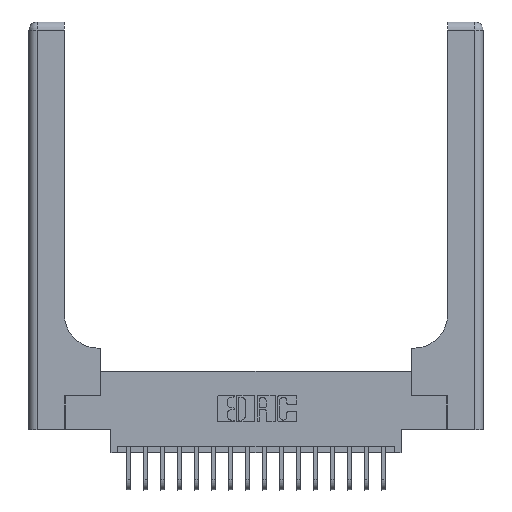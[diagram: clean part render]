
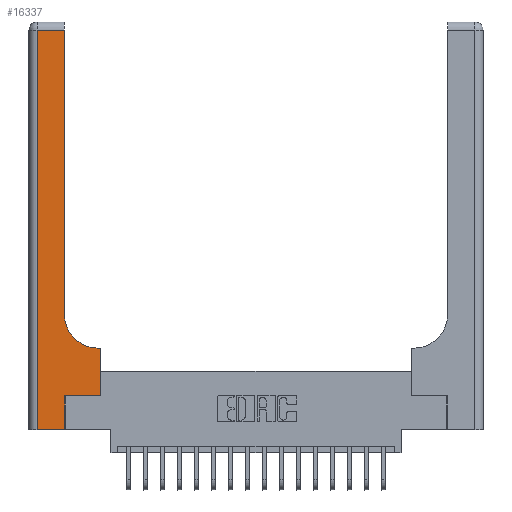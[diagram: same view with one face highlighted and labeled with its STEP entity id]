
A CAD part, top view. The second image highlights one B-rep face of the part: STEP entity #16337.
In plain terms, the highlighted planar face has unit normal (0, 0, 1).
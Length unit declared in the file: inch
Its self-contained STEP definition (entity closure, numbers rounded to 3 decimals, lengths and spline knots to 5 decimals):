
#122 = VECTOR ( 'NONE', #10542, 39.37008 ) ;
#211 = VERTEX_POINT ( 'NONE', #7665 ) ;
#335 = ORIENTED_EDGE ( 'NONE', *, *, #12892, .T. ) ;
#625 = DIRECTION ( 'NONE',  ( 0., 0., -1. ) ) ;
#673 = CARTESIAN_POINT ( 'NONE',  ( 0.265, 0., 0.37 ) ) ;
#1285 = EDGE_CURVE ( 'NONE', #3510, #17253, #9000, .T. ) ;
#1642 = AXIS2_PLACEMENT_3D ( 'NONE', #3078, #9773, #6152 ) ;
#1792 = LINE ( 'NONE', #16711, #8638 ) ;
#2145 = CARTESIAN_POINT ( 'NONE',  ( 0.528, 0.25, 0.37 ) ) ;
#2378 = LINE ( 'NONE', #12741, #17226 ) ;
#2574 = EDGE_CURVE ( 'NONE', #4467, #6856, #1792, .T. ) ;
#2607 = ORIENTED_EDGE ( 'NONE', *, *, #15406, .T. ) ;
#2895 = CARTESIAN_POINT ( 'NONE',  ( 0.265, 0.25, 0.37 ) ) ;
#3078 = CARTESIAN_POINT ( 'NONE',  ( 0.51, 0.85, 0.37 ) ) ;
#3272 = AXIS2_PLACEMENT_3D ( 'NONE', #15536, #625, #7302 ) ;
#3510 = VERTEX_POINT ( 'NONE', #9975 ) ;
#3886 = PLANE ( 'NONE',  #3272 ) ;
#3890 = ORIENTED_EDGE ( 'NONE', *, *, #6887, .T. ) ;
#4261 = CARTESIAN_POINT ( 'NONE',  ( 0.06, 3., 0.37 ) ) ;
#4445 = VERTEX_POINT ( 'NONE', #673 ) ;
#4467 = VERTEX_POINT ( 'NONE', #20370 ) ;
#5089 = DIRECTION ( 'NONE',  ( -1., 0., 0. ) ) ;
#6149 = CARTESIAN_POINT ( 'NONE',  ( 0.265, 0.25, 0.37 ) ) ;
#6152 = DIRECTION ( 'NONE',  ( 1., 0., 0. ) ) ;
#6190 = ORIENTED_EDGE ( 'NONE', *, *, #1285, .T. ) ;
#6856 = VERTEX_POINT ( 'NONE', #17533 ) ;
#6887 = EDGE_CURVE ( 'NONE', #6856, #15495, #11058, .T. ) ;
#7302 = DIRECTION ( 'NONE',  ( -1., 0., 0. ) ) ;
#7633 = VECTOR ( 'NONE', #19273, 39.37008 ) ;
#7665 = CARTESIAN_POINT ( 'NONE',  ( 0.26, 2.94, 0.37 ) ) ;
#7694 = LINE ( 'NONE', #16035, #7739 ) ;
#7739 = VECTOR ( 'NONE', #11409, 39.37008 ) ;
#7845 = ORIENTED_EDGE ( 'NONE', *, *, #11887, .T. ) ;
#8092 = DIRECTION ( 'NONE',  ( 0., 1., 0. ) ) ;
#8638 = VECTOR ( 'NONE', #5089, 39.37008 ) ;
#9000 = LINE ( 'NONE', #4261, #7633 ) ;
#9269 = FACE_OUTER_BOUND ( 'NONE', #9781, .T. ) ;
#9612 = VECTOR ( 'NONE', #18584, 39.37008 ) ;
#9737 = LINE ( 'NONE', #17942, #12927 ) ;
#9773 = DIRECTION ( 'NONE',  ( 0., 0., -1. ) ) ;
#9781 = EDGE_LOOP ( 'NONE', ( #10367, #12517, #6190, #7845, #335, #18837, #2607, #13798, #3890 ) ) ;
#9880 = CARTESIAN_POINT ( 'NONE',  ( 0., 2.94, 0.37 ) ) ;
#9975 = CARTESIAN_POINT ( 'NONE',  ( 0.06, 2.94, 0.37 ) ) ;
#10367 = ORIENTED_EDGE ( 'NONE', *, *, #18228, .T. ) ;
#10542 = DIRECTION ( 'NONE',  ( 0., 1., 0. ) ) ;
#11058 = CIRCLE ( 'NONE', #1642, 0.25 ) ;
#11409 = DIRECTION ( 'NONE',  ( 1., 0., 0. ) ) ;
#11603 = LINE ( 'NONE', #9880, #9612 ) ;
#11887 = EDGE_CURVE ( 'NONE', #17253, #4445, #7694, .T. ) ;
#12517 = ORIENTED_EDGE ( 'NONE', *, *, #17177, .T. ) ;
#12741 = CARTESIAN_POINT ( 'NONE',  ( 0.26, 3., 0.37 ) ) ;
#12892 = EDGE_CURVE ( 'NONE', #4445, #19646, #9737, .T. ) ;
#12927 = VECTOR ( 'NONE', #8092, 39.37008 ) ;
#12944 = DIRECTION ( 'NONE',  ( 1., 0., 0. ) ) ;
#13798 = ORIENTED_EDGE ( 'NONE', *, *, #2574, .T. ) ;
#14722 = CARTESIAN_POINT ( 'NONE',  ( 0.26, 0.85, 0.37 ) ) ;
#14725 = CARTESIAN_POINT ( 'NONE',  ( 0.06, 0., 0.37 ) ) ;
#15298 = LINE ( 'NONE', #17136, #122 ) ;
#15406 = EDGE_CURVE ( 'NONE', #21186, #4467, #15298, .T. ) ;
#15495 = VERTEX_POINT ( 'NONE', #14722 ) ;
#15536 = CARTESIAN_POINT ( 'NONE',  ( 0., 3., 0.37 ) ) ;
#16035 = CARTESIAN_POINT ( 'NONE',  ( 0., 0., 0.37 ) ) ;
#16337 = ADVANCED_FACE ( 'NONE', ( #9269 ), #3886, .F. ) ;
#16711 = CARTESIAN_POINT ( 'NONE',  ( 0.26, 0.6, 0.37 ) ) ;
#17136 = CARTESIAN_POINT ( 'NONE',  ( 0.528, 0.25, 0.37 ) ) ;
#17177 = EDGE_CURVE ( 'NONE', #211, #3510, #11603, .T. ) ;
#17226 = VECTOR ( 'NONE', #19351, 39.37008 ) ;
#17253 = VERTEX_POINT ( 'NONE', #14725 ) ;
#17533 = CARTESIAN_POINT ( 'NONE',  ( 0.51, 0.6, 0.37 ) ) ;
#17942 = CARTESIAN_POINT ( 'NONE',  ( 0.265, 0., 0.37 ) ) ;
#18228 = EDGE_CURVE ( 'NONE', #15495, #211, #2378, .T. ) ;
#18584 = DIRECTION ( 'NONE',  ( -1., 0., 0. ) ) ;
#18733 = EDGE_CURVE ( 'NONE', #19646, #21186, #19433, .T. ) ;
#18837 = ORIENTED_EDGE ( 'NONE', *, *, #18733, .T. ) ;
#19273 = DIRECTION ( 'NONE',  ( 0., -1., 0. ) ) ;
#19351 = DIRECTION ( 'NONE',  ( 0., 1., 0. ) ) ;
#19433 = LINE ( 'NONE', #2895, #20360 ) ;
#19646 = VERTEX_POINT ( 'NONE', #6149 ) ;
#20360 = VECTOR ( 'NONE', #12944, 39.37008 ) ;
#20370 = CARTESIAN_POINT ( 'NONE',  ( 0.528, 0.6, 0.37 ) ) ;
#21186 = VERTEX_POINT ( 'NONE', #2145 ) ;
